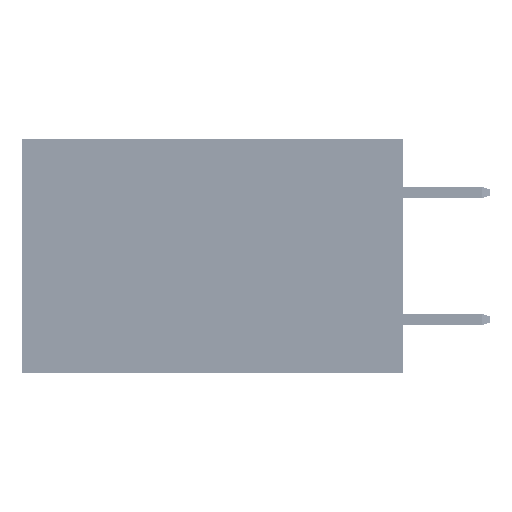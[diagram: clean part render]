
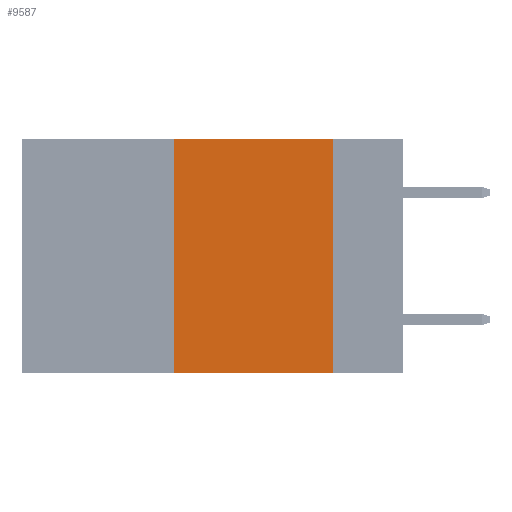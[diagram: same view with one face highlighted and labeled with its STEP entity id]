
A CAD part, left-side view. The second image highlights one B-rep face of the part: STEP entity #9587.
In plain terms, the highlighted planar face has unit normal (-1, 0, 0).
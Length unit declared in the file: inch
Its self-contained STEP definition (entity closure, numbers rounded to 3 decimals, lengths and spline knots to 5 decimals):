
#1044 = DIRECTION ( 'NONE',  ( 0., -1., 0. ) ) ;
#1627 = VERTEX_POINT ( 'NONE', #23889 ) ;
#2492 = VECTOR ( 'NONE', #1044, 39.37008 ) ;
#3122 = ORIENTED_EDGE ( 'NONE', *, *, #6014, .F. ) ;
#3157 = PLANE ( 'NONE',  #33488 ) ;
#3410 = FACE_OUTER_BOUND ( 'NONE', #7896, .T. ) ;
#3983 = VERTEX_POINT ( 'NONE', #30981 ) ;
#4312 = CARTESIAN_POINT ( 'NONE',  ( 0., 0.11, 0. ) ) ;
#6014 = EDGE_CURVE ( 'NONE', #3983, #37376, #11653, .T. ) ;
#7525 = DIRECTION ( 'NONE',  ( 0., -1., 0. ) ) ;
#7807 = DIRECTION ( 'NONE',  ( 0., 0., 1. ) ) ;
#7896 = EDGE_LOOP ( 'NONE', ( #21127, #9384, #3122, #25410 ) ) ;
#9384 = ORIENTED_EDGE ( 'NONE', *, *, #31723, .F. ) ;
#9587 = ADVANCED_FACE ( 'NONE', ( #3410 ), #3157, .F. ) ;
#11653 = LINE ( 'NONE', #23710, #20276 ) ;
#17854 = VECTOR ( 'NONE', #36121, 39.37008 ) ;
#18832 = CARTESIAN_POINT ( 'NONE',  ( 0., 0.11, 0. ) ) ;
#19064 = CARTESIAN_POINT ( 'NONE',  ( 0., 0.6, 0. ) ) ;
#20276 = VECTOR ( 'NONE', #7807, 39.37008 ) ;
#21127 = ORIENTED_EDGE ( 'NONE', *, *, #34023, .F. ) ;
#21415 = VECTOR ( 'NONE', #7525, 39.37008 ) ;
#23710 = CARTESIAN_POINT ( 'NONE',  ( 0., 0.36, 0. ) ) ;
#23889 = CARTESIAN_POINT ( 'NONE',  ( 0., 0.11, -0.37 ) ) ;
#24643 = LINE ( 'NONE', #47719, #2492 ) ;
#25410 = ORIENTED_EDGE ( 'NONE', *, *, #38907, .T. ) ;
#28565 = VERTEX_POINT ( 'NONE', #18832 ) ;
#30981 = CARTESIAN_POINT ( 'NONE',  ( 0., 0.36, -0.37 ) ) ;
#31127 = LINE ( 'NONE', #38056, #21415 ) ;
#31723 = EDGE_CURVE ( 'NONE', #37376, #28565, #31127, .T. ) ;
#32266 = CARTESIAN_POINT ( 'NONE',  ( 0., 0.36, 0. ) ) ;
#33488 = AXIS2_PLACEMENT_3D ( 'NONE', #19064, #38301, #33946 ) ;
#33946 = DIRECTION ( 'NONE',  ( 0., 0., -1. ) ) ;
#34023 = EDGE_CURVE ( 'NONE', #28565, #1627, #43817, .T. ) ;
#36121 = DIRECTION ( 'NONE',  ( 0., 0., -1. ) ) ;
#37376 = VERTEX_POINT ( 'NONE', #32266 ) ;
#38056 = CARTESIAN_POINT ( 'NONE',  ( 0., 0.6, 0. ) ) ;
#38301 = DIRECTION ( 'NONE',  ( 1., 0., 0. ) ) ;
#38907 = EDGE_CURVE ( 'NONE', #3983, #1627, #24643, .T. ) ;
#43817 = LINE ( 'NONE', #4312, #17854 ) ;
#47719 = CARTESIAN_POINT ( 'NONE',  ( 0., 0.6, -0.37 ) ) ;
